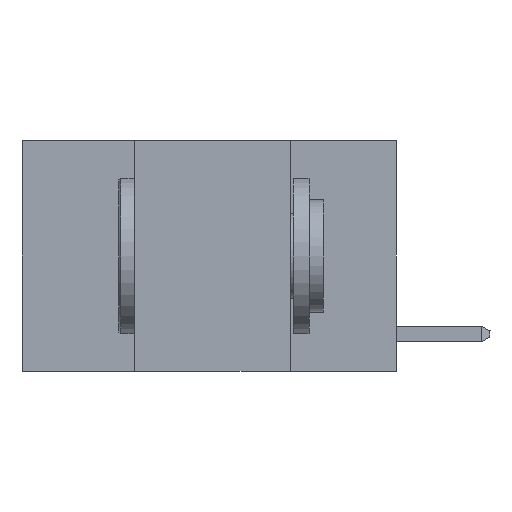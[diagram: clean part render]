
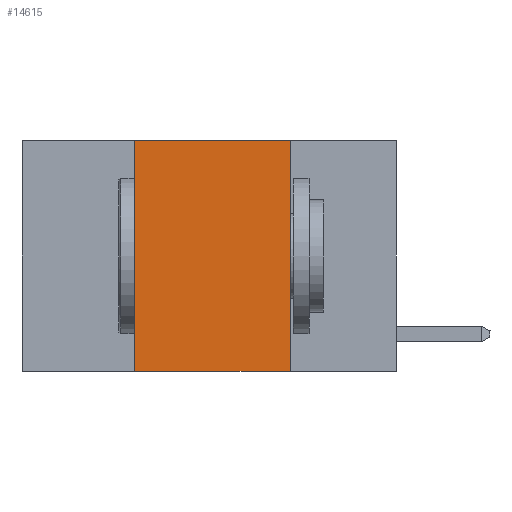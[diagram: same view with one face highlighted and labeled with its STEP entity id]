
A CAD part, left-side view. The second image highlights one B-rep face of the part: STEP entity #14615.
In plain terms, the highlighted planar face has unit normal (-1, 0, 0).
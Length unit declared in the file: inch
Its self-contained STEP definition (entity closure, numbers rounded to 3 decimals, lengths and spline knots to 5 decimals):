
#405 = EDGE_CURVE ( 'NONE', #8887, #19099, #5069, .T. ) ;
#2294 = DIRECTION ( 'NONE',  ( 0., 0., -1. ) ) ;
#3176 = CARTESIAN_POINT ( 'NONE',  ( 0., 0.6, -0.37 ) ) ;
#3521 = VECTOR ( 'NONE', #15521, 39.37008 ) ;
#3657 = CARTESIAN_POINT ( 'NONE',  ( 0., 0.42, 0. ) ) ;
#4229 = AXIS2_PLACEMENT_3D ( 'NONE', #8217, #11901, #2294 ) ;
#4412 = PLANE ( 'NONE',  #4229 ) ;
#4662 = FACE_OUTER_BOUND ( 'NONE', #11806, .T. ) ;
#4805 = CARTESIAN_POINT ( 'NONE',  ( 0., 0.17, 0. ) ) ;
#5040 = LINE ( 'NONE', #18816, #14170 ) ;
#5069 = LINE ( 'NONE', #9500, #3521 ) ;
#5670 = EDGE_CURVE ( 'NONE', #17170, #8887, #15008, .T. ) ;
#8217 = CARTESIAN_POINT ( 'NONE',  ( 0., 0.6, 0. ) ) ;
#8532 = ORIENTED_EDGE ( 'NONE', *, *, #405, .F. ) ;
#8887 = VERTEX_POINT ( 'NONE', #3657 ) ;
#9500 = CARTESIAN_POINT ( 'NONE',  ( 0., 0.6, 0. ) ) ;
#11783 = EDGE_CURVE ( 'NONE', #17170, #17432, #12717, .T. ) ;
#11806 = EDGE_LOOP ( 'NONE', ( #20898, #8532, #14629, #24492 ) ) ;
#11901 = DIRECTION ( 'NONE',  ( 1., 0., 0. ) ) ;
#12717 = LINE ( 'NONE', #3176, #18907 ) ;
#14170 = VECTOR ( 'NONE', #17139, 39.37008 ) ;
#14615 = ADVANCED_FACE ( 'NONE', ( #4662 ), #4412, .F. ) ;
#14629 = ORIENTED_EDGE ( 'NONE', *, *, #5670, .F. ) ;
#15008 = LINE ( 'NONE', #25081, #21840 ) ;
#15521 = DIRECTION ( 'NONE',  ( 0., -1., 0. ) ) ;
#17139 = DIRECTION ( 'NONE',  ( 0., 0., -1. ) ) ;
#17170 = VERTEX_POINT ( 'NONE', #23293 ) ;
#17432 = VERTEX_POINT ( 'NONE', #24141 ) ;
#18816 = CARTESIAN_POINT ( 'NONE',  ( 0., 0.17, 0. ) ) ;
#18888 = DIRECTION ( 'NONE',  ( 0., -1., 0. ) ) ;
#18907 = VECTOR ( 'NONE', #18888, 39.37008 ) ;
#19099 = VERTEX_POINT ( 'NONE', #4805 ) ;
#20898 = ORIENTED_EDGE ( 'NONE', *, *, #22312, .F. ) ;
#21840 = VECTOR ( 'NONE', #22952, 39.37008 ) ;
#22312 = EDGE_CURVE ( 'NONE', #19099, #17432, #5040, .T. ) ;
#22952 = DIRECTION ( 'NONE',  ( 0., 0., 1. ) ) ;
#23293 = CARTESIAN_POINT ( 'NONE',  ( 0., 0.42, -0.37 ) ) ;
#24141 = CARTESIAN_POINT ( 'NONE',  ( 0., 0.17, -0.37 ) ) ;
#24492 = ORIENTED_EDGE ( 'NONE', *, *, #11783, .T. ) ;
#25081 = CARTESIAN_POINT ( 'NONE',  ( 0., 0.42, 0. ) ) ;
